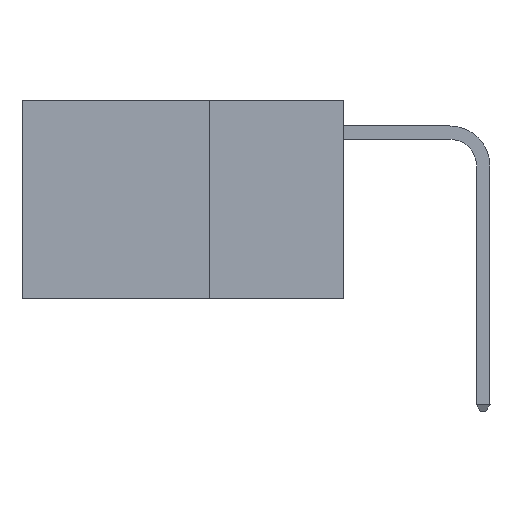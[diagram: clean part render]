
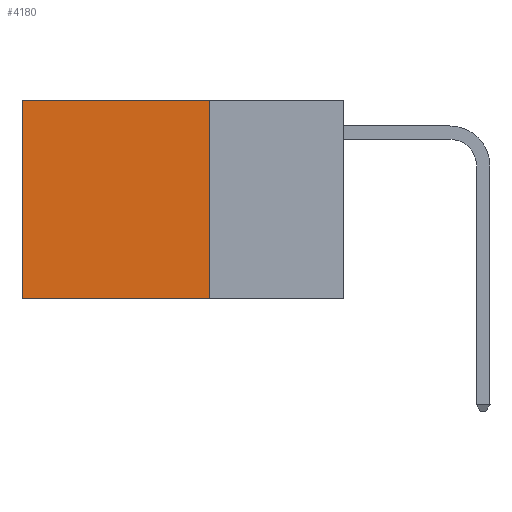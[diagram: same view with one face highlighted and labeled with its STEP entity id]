
A CAD part, left-side view. The second image highlights one B-rep face of the part: STEP entity #4180.
In plain terms, the highlighted planar face has unit normal (-1, 0, 0).
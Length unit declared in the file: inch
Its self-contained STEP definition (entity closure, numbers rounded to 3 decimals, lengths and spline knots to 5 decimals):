
#2757 = LINE ( 'NONE', #2811, #13453 ) ;
#2811 = CARTESIAN_POINT ( 'NONE',  ( 0.2625, 0.25, -0.37 ) ) ;
#3633 = VECTOR ( 'NONE', #7314, 39.37008 ) ;
#4120 = VERTEX_POINT ( 'NONE', #13919 ) ;
#4180 = ADVANCED_FACE ( 'NONE', ( #16244 ), #12722, .F. ) ;
#4488 = ORIENTED_EDGE ( 'NONE', *, *, #16644, .F. ) ;
#4794 = DIRECTION ( 'NONE',  ( 1., 0., 0. ) ) ;
#5637 = DIRECTION ( 'NONE',  ( 0., 1., 0. ) ) ;
#6024 = AXIS2_PLACEMENT_3D ( 'NONE', #8796, #4794, #14027 ) ;
#6831 = VECTOR ( 'NONE', #7075, 39.37008 ) ;
#6946 = VERTEX_POINT ( 'NONE', #9345 ) ;
#7075 = DIRECTION ( 'NONE',  ( 0., 1., 0. ) ) ;
#7314 = DIRECTION ( 'NONE',  ( 0., 0., -1. ) ) ;
#7323 = ORIENTED_EDGE ( 'NONE', *, *, #8559, .T. ) ;
#8111 = VERTEX_POINT ( 'NONE', #15764 ) ;
#8156 = EDGE_CURVE ( 'NONE', #15348, #6946, #16887, .T. ) ;
#8559 = EDGE_CURVE ( 'NONE', #8111, #4120, #9983, .T. ) ;
#8796 = CARTESIAN_POINT ( 'NONE',  ( 0.2625, 0.25, 0. ) ) ;
#9345 = CARTESIAN_POINT ( 'NONE',  ( 0.2625, 0.25, -0.37 ) ) ;
#9634 = ORIENTED_EDGE ( 'NONE', *, *, #8156, .F. ) ;
#9925 = LINE ( 'NONE', #14904, #6831 ) ;
#9983 = LINE ( 'NONE', #15118, #3633 ) ;
#10262 = EDGE_CURVE ( 'NONE', #15348, #8111, #9925, .T. ) ;
#12722 = PLANE ( 'NONE',  #6024 ) ;
#12733 = CARTESIAN_POINT ( 'NONE',  ( 0.2625, 0.25, 0. ) ) ;
#12782 = ORIENTED_EDGE ( 'NONE', *, *, #10262, .T. ) ;
#13049 = VECTOR ( 'NONE', #13300, 39.37008 ) ;
#13120 = EDGE_LOOP ( 'NONE', ( #7323, #4488, #9634, #12782 ) ) ;
#13300 = DIRECTION ( 'NONE',  ( 0., 0., -1. ) ) ;
#13453 = VECTOR ( 'NONE', #5637, 39.37008 ) ;
#13919 = CARTESIAN_POINT ( 'NONE',  ( 0.2625, 0.6, -0.37 ) ) ;
#14027 = DIRECTION ( 'NONE',  ( 0., 0., -1. ) ) ;
#14904 = CARTESIAN_POINT ( 'NONE',  ( 0.2625, 0.25, 0. ) ) ;
#15118 = CARTESIAN_POINT ( 'NONE',  ( 0.2625, 0.6, 0. ) ) ;
#15348 = VERTEX_POINT ( 'NONE', #12733 ) ;
#15764 = CARTESIAN_POINT ( 'NONE',  ( 0.2625, 0.6, 0. ) ) ;
#16244 = FACE_OUTER_BOUND ( 'NONE', #13120, .T. ) ;
#16644 = EDGE_CURVE ( 'NONE', #6946, #4120, #2757, .T. ) ;
#16887 = LINE ( 'NONE', #17082, #13049 ) ;
#17082 = CARTESIAN_POINT ( 'NONE',  ( 0.2625, 0.25, 0. ) ) ;
